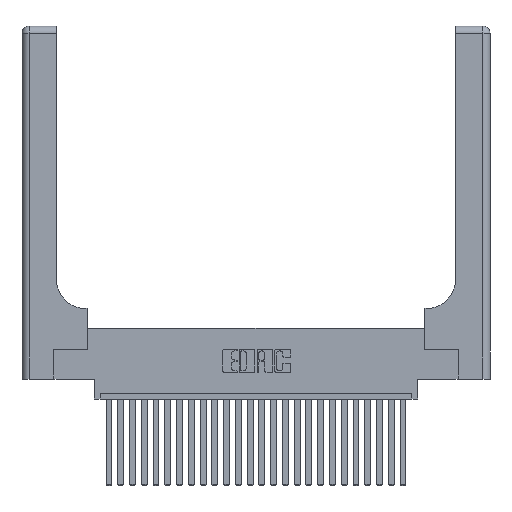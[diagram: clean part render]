
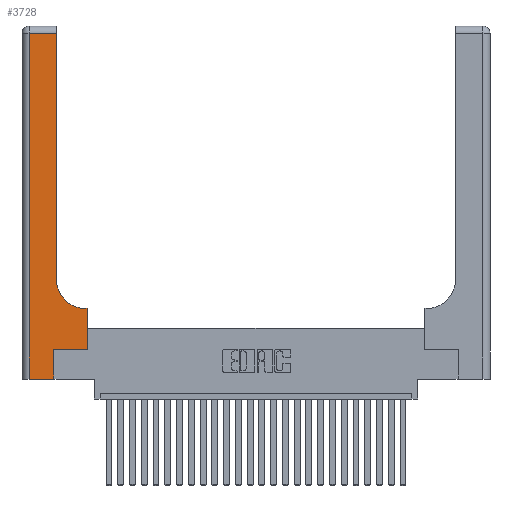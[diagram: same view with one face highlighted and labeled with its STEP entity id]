
A CAD part, top view. The second image highlights one B-rep face of the part: STEP entity #3728.
In plain terms, the highlighted planar face has unit normal (0, 0, 1).
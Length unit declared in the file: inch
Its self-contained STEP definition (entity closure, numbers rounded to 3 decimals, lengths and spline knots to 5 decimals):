
#9 = VERTEX_POINT ( 'NONE', #16914 ) ;
#174 = LINE ( 'NONE', #10225, #20940 ) ;
#669 = CARTESIAN_POINT ( 'NONE',  ( 0.5585, 0.25, 0.37 ) ) ;
#887 = EDGE_CURVE ( 'NONE', #22931, #18744, #20082, .T. ) ;
#1295 = CARTESIAN_POINT ( 'NONE',  ( 0.269, 0., 0.37 ) ) ;
#1775 = CARTESIAN_POINT ( 'NONE',  ( 0.06, 2.94, 0.37 ) ) ;
#3499 = LINE ( 'NONE', #669, #11219 ) ;
#3708 = CARTESIAN_POINT ( 'NONE',  ( 0.269, 0., 0.37 ) ) ;
#3728 = ADVANCED_FACE ( 'NONE', ( #24713 ), #24385, .F. ) ;
#4716 = ORIENTED_EDGE ( 'NONE', *, *, #10868, .T. ) ;
#4877 = CARTESIAN_POINT ( 'NONE',  ( 0., 0., 0.37 ) ) ;
#5258 = VECTOR ( 'NONE', #19584, 39.37008 ) ;
#5307 = CARTESIAN_POINT ( 'NONE',  ( 0.06, 3., 0.37 ) ) ;
#5790 = DIRECTION ( 'NONE',  ( -1., 0., 0. ) ) ;
#6797 = CARTESIAN_POINT ( 'NONE',  ( 0.2915, 3., 0.37 ) ) ;
#6845 = LINE ( 'NONE', #4877, #5258 ) ;
#7372 = DIRECTION ( 'NONE',  ( 0., -1., 0. ) ) ;
#7663 = VECTOR ( 'NONE', #18902, 39.37008 ) ;
#8300 = CARTESIAN_POINT ( 'NONE',  ( 0.2915, 0.85, 0.37 ) ) ;
#8459 = DIRECTION ( 'NONE',  ( -1., 0., 0. ) ) ;
#8485 = EDGE_CURVE ( 'NONE', #18744, #18003, #25147, .T. ) ;
#8752 = DIRECTION ( 'NONE',  ( 1., 0., 0. ) ) ;
#9160 = CARTESIAN_POINT ( 'NONE',  ( 0.5585, 0.6, 0.37 ) ) ;
#10225 = CARTESIAN_POINT ( 'NONE',  ( 0.269, 0.25, 0.37 ) ) ;
#10283 = CARTESIAN_POINT ( 'NONE',  ( 0., 2.94, 0.37 ) ) ;
#10791 = ORIENTED_EDGE ( 'NONE', *, *, #23259, .T. ) ;
#10868 = EDGE_CURVE ( 'NONE', #25909, #22931, #16389, .T. ) ;
#10962 = LINE ( 'NONE', #17669, #23340 ) ;
#11219 = VECTOR ( 'NONE', #17119, 39.37008 ) ;
#11366 = ORIENTED_EDGE ( 'NONE', *, *, #17191, .T. ) ;
#11614 = ORIENTED_EDGE ( 'NONE', *, *, #26001, .T. ) ;
#12000 = CARTESIAN_POINT ( 'NONE',  ( 0.5415, 0.85, 0.37 ) ) ;
#12785 = VERTEX_POINT ( 'NONE', #13309 ) ;
#13309 = CARTESIAN_POINT ( 'NONE',  ( 0.5585, 0.25, 0.37 ) ) ;
#13339 = EDGE_CURVE ( 'NONE', #18003, #20039, #6845, .T. ) ;
#14632 = EDGE_LOOP ( 'NONE', ( #4716, #26835, #25369, #23231, #15812, #11614, #11366, #10791, #17544 ) ) ;
#15426 = CARTESIAN_POINT ( 'NONE',  ( 0.5415, 0.6, 0.37 ) ) ;
#15812 = ORIENTED_EDGE ( 'NONE', *, *, #24156, .T. ) ;
#16180 = DIRECTION ( 'NONE',  ( 0., 0., -1. ) ) ;
#16363 = DIRECTION ( 'NONE',  ( 1., 0., 0. ) ) ;
#16389 = LINE ( 'NONE', #6797, #22559 ) ;
#16914 = CARTESIAN_POINT ( 'NONE',  ( 0.269, 0.25, 0.37 ) ) ;
#17119 = DIRECTION ( 'NONE',  ( 0., 1., 0. ) ) ;
#17191 = EDGE_CURVE ( 'NONE', #12785, #22718, #3499, .T. ) ;
#17437 = AXIS2_PLACEMENT_3D ( 'NONE', #22199, #26398, #5790 ) ;
#17544 = ORIENTED_EDGE ( 'NONE', *, *, #24079, .T. ) ;
#17669 = CARTESIAN_POINT ( 'NONE',  ( 0.2915, 0.6, 0.37 ) ) ;
#18003 = VERTEX_POINT ( 'NONE', #20216 ) ;
#18436 = VERTEX_POINT ( 'NONE', #15426 ) ;
#18744 = VERTEX_POINT ( 'NONE', #1775 ) ;
#18902 = DIRECTION ( 'NONE',  ( 0., 1., 0. ) ) ;
#19584 = DIRECTION ( 'NONE',  ( 1., 0., 0. ) ) ;
#19847 = AXIS2_PLACEMENT_3D ( 'NONE', #12000, #16180, #16363 ) ;
#20039 = VERTEX_POINT ( 'NONE', #1295 ) ;
#20082 = LINE ( 'NONE', #10283, #26597 ) ;
#20216 = CARTESIAN_POINT ( 'NONE',  ( 0.06, 0., 0.37 ) ) ;
#20940 = VECTOR ( 'NONE', #8752, 39.37008 ) ;
#21238 = VECTOR ( 'NONE', #7372, 39.37008 ) ;
#22199 = CARTESIAN_POINT ( 'NONE',  ( 0., 3., 0.37 ) ) ;
#22559 = VECTOR ( 'NONE', #25969, 39.37008 ) ;
#22718 = VERTEX_POINT ( 'NONE', #9160 ) ;
#22931 = VERTEX_POINT ( 'NONE', #26619 ) ;
#23231 = ORIENTED_EDGE ( 'NONE', *, *, #13339, .T. ) ;
#23259 = EDGE_CURVE ( 'NONE', #22718, #18436, #10962, .T. ) ;
#23340 = VECTOR ( 'NONE', #23933, 39.37008 ) ;
#23933 = DIRECTION ( 'NONE',  ( -1., 0., 0. ) ) ;
#24079 = EDGE_CURVE ( 'NONE', #18436, #25909, #25234, .T. ) ;
#24156 = EDGE_CURVE ( 'NONE', #20039, #9, #26210, .T. ) ;
#24385 = PLANE ( 'NONE',  #17437 ) ;
#24713 = FACE_OUTER_BOUND ( 'NONE', #14632, .T. ) ;
#25147 = LINE ( 'NONE', #5307, #21238 ) ;
#25234 = CIRCLE ( 'NONE', #19847, 0.25 ) ;
#25369 = ORIENTED_EDGE ( 'NONE', *, *, #8485, .T. ) ;
#25909 = VERTEX_POINT ( 'NONE', #8300 ) ;
#25969 = DIRECTION ( 'NONE',  ( 0., 1., 0. ) ) ;
#26001 = EDGE_CURVE ( 'NONE', #9, #12785, #174, .T. ) ;
#26210 = LINE ( 'NONE', #3708, #7663 ) ;
#26398 = DIRECTION ( 'NONE',  ( 0., 0., -1. ) ) ;
#26597 = VECTOR ( 'NONE', #8459, 39.37008 ) ;
#26619 = CARTESIAN_POINT ( 'NONE',  ( 0.2915, 2.94, 0.37 ) ) ;
#26835 = ORIENTED_EDGE ( 'NONE', *, *, #887, .T. ) ;
